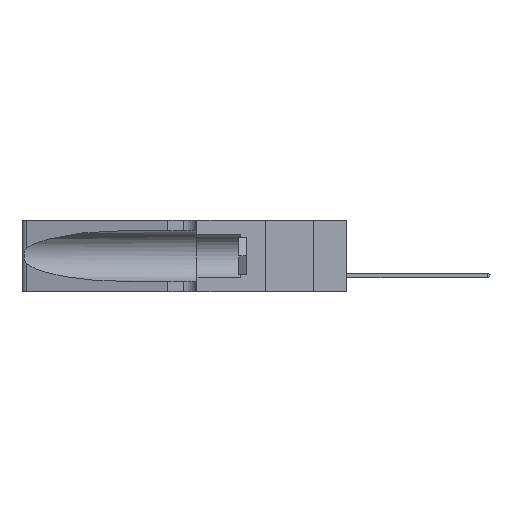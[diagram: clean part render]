
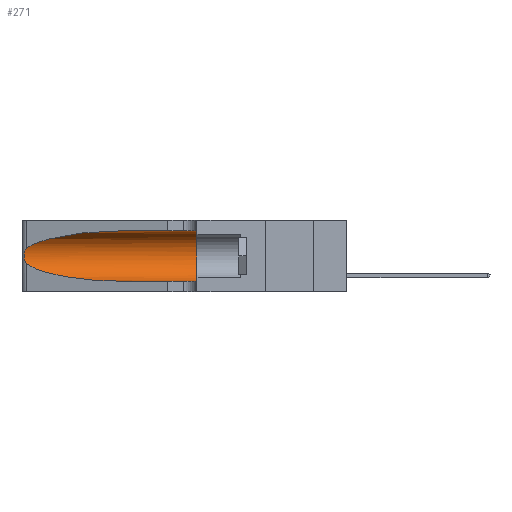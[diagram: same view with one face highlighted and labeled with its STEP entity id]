
A CAD part, left-side view. The second image highlights one B-rep face of the part: STEP entity #271.
In plain terms, the highlighted cylindrical face has radius 3.308 mm (diameter 6.617 mm), a partial arc.
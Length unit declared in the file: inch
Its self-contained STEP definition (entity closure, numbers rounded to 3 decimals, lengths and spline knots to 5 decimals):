
#271 = ADVANCED_FACE ( 'NONE', ( #20561 ), #32296, .F. ) ;
#334 = VERTEX_POINT ( 'NONE', #22993 ) ;
#437 = EDGE_LOOP ( 'NONE', ( #36061, #23964, #4984, #29937, #17057, #5986 ) ) ;
#499 = DIRECTION ( 'NONE',  ( 0., -1., 0. ) ) ;
#3479 = VERTEX_POINT ( 'NONE', #29351 ) ;
#3822 = LINE ( 'NONE', #5627, #8558 ) ;
#3956 = CARTESIAN_POINT ( 'NONE',  ( 0.26075, 1.23896, 0.178 ) ) ;
#3970 = CARTESIAN_POINT ( 'NONE',  ( 0.18966, 0.96281, 0.05475 ) ) ;
#4095 = CARTESIAN_POINT ( 'NONE',  ( 0.26075, 1.23896, 0.19203 ) ) ;
#4477 = CARTESIAN_POINT ( 'NONE',  ( 0.25487, 1.22718, 0.22369 ) ) ;
#4726 = EDGE_CURVE ( 'NONE', #3479, #27880, #16341, .T. ) ;
#4984 = ORIENTED_EDGE ( 'NONE', *, *, #6401, .T. ) ;
#5206 = VERTEX_POINT ( 'NONE', #27979 ) ;
#5441 = B_SPLINE_CURVE_WITH_KNOTS ( 'NONE', 3,
 ( #32488, #29800, #38594, #38480, #18253, #21294, #4095, #3956, #30803, #10031, #19609, #34381, #37412, #28608 ),
 .UNSPECIFIED., .F., .F.,
 ( 4, 2, 2, 2, 2, 2, 4 ),
 ( 0., 0.00027, 0.00053, 0.00107, 0.0016, 0.00187, 0.00214 ),
 .UNSPECIFIED. ) ;
#5627 = CARTESIAN_POINT ( 'NONE',  ( 0.1305, 1.61858, 0.31525 ) ) ;
#5986 = ORIENTED_EDGE ( 'NONE', *, *, #37150, .F. ) ;
#6135 = AXIS2_PLACEMENT_3D ( 'NONE', #24913, #18904, #18771 ) ;
#6401 = EDGE_CURVE ( 'NONE', #32020, #29624, #7006, .T. ) ;
#7006 =( BOUNDED_CURVE ( )  B_SPLINE_CURVE ( 3, ( #28217, #18804, #3970, #33987 ),
 .UNSPECIFIED., .F., .F. ) 
 B_SPLINE_CURVE_WITH_KNOTS ( ( 4, 4 ),
 ( 3.44316, 4.71239 ),
 .UNSPECIFIED. ) 
 CURVE ( )  GEOMETRIC_REPRESENTATION_ITEM ( )  RATIONAL_B_SPLINE_CURVE ( ( 1., 0.87, 0.87, 1. ) ) 
 REPRESENTATION_ITEM ( '' )  );
#7859 = CARTESIAN_POINT ( 'NONE',  ( 0.25487, 1.22718, 0.22369 ) ) ;
#8558 = VECTOR ( 'NONE', #35507, 39.37008 ) ;
#10031 = CARTESIAN_POINT ( 'NONE',  ( 0.25856, 1.23593, 0.16098 ) ) ;
#15086 = CARTESIAN_POINT ( 'NONE',  ( 0.1305, 1.61858, 0.185 ) ) ;
#15327 = DIRECTION ( 'NONE',  ( 0., 0., -1. ) ) ;
#16226 = CARTESIAN_POINT ( 'NONE',  ( 0.25487, 1.22718, 0.14631 ) ) ;
#16341 =( BOUNDED_CURVE ( )  B_SPLINE_CURVE ( 3, ( #28430, #34614, #19999, #7859 ),
 .UNSPECIFIED., .F., .F. ) 
 B_SPLINE_CURVE_WITH_KNOTS ( ( 4, 4 ),
 ( 1.5708, 2.84003 ),
 .UNSPECIFIED. ) 
 CURVE ( )  GEOMETRIC_REPRESENTATION_ITEM ( )  RATIONAL_B_SPLINE_CURVE ( ( 1., 0.87, 0.87, 1. ) ) 
 REPRESENTATION_ITEM ( '' )  );
#16529 = CARTESIAN_POINT ( 'NONE',  ( 0.1305, 0.72297, 0.05475 ) ) ;
#17057 = ORIENTED_EDGE ( 'NONE', *, *, #36085, .F. ) ;
#18253 = CARTESIAN_POINT ( 'NONE',  ( 0.25854, 1.2359, 0.20912 ) ) ;
#18771 = DIRECTION ( 'NONE',  ( 0., 0., 1. ) ) ;
#18804 = CARTESIAN_POINT ( 'NONE',  ( 0.2373, 1.15595, 0.08982 ) ) ;
#18904 = DIRECTION ( 'NONE',  ( 0., 1., 0. ) ) ;
#19235 = CIRCLE ( 'NONE', #6135, 0.13025 ) ;
#19609 = CARTESIAN_POINT ( 'NONE',  ( 0.25789, 1.23486, 0.15765 ) ) ;
#19999 = CARTESIAN_POINT ( 'NONE',  ( 0.2373, 1.15595, 0.28018 ) ) ;
#20561 = FACE_OUTER_BOUND ( 'NONE', #437, .T. ) ;
#21294 = CARTESIAN_POINT ( 'NONE',  ( 0.26018, 1.23835, 0.19895 ) ) ;
#22984 = VECTOR ( 'NONE', #36687, 39.37008 ) ;
#22993 = CARTESIAN_POINT ( 'NONE',  ( 0.1305, 0.35, 0.05475 ) ) ;
#23964 = ORIENTED_EDGE ( 'NONE', *, *, #24600, .T. ) ;
#24600 = EDGE_CURVE ( 'NONE', #27880, #32020, #5441, .T. ) ;
#24913 = CARTESIAN_POINT ( 'NONE',  ( 0.1305, 0.35, 0.185 ) ) ;
#27880 = VERTEX_POINT ( 'NONE', #4477 ) ;
#27979 = CARTESIAN_POINT ( 'NONE',  ( 0.1305, 0.35, 0.31525 ) ) ;
#28202 = AXIS2_PLACEMENT_3D ( 'NONE', #15086, #499, #15327 ) ;
#28217 = CARTESIAN_POINT ( 'NONE',  ( 0.25487, 1.22718, 0.14631 ) ) ;
#28430 = CARTESIAN_POINT ( 'NONE',  ( 0.1305, 0.72297, 0.31525 ) ) ;
#28608 = CARTESIAN_POINT ( 'NONE',  ( 0.25487, 1.22718, 0.14631 ) ) ;
#29351 = CARTESIAN_POINT ( 'NONE',  ( 0.1305, 0.72297, 0.31525 ) ) ;
#29624 = VERTEX_POINT ( 'NONE', #16529 ) ;
#29800 = CARTESIAN_POINT ( 'NONE',  ( 0.25555, 1.22994, 0.2215 ) ) ;
#29937 = ORIENTED_EDGE ( 'NONE', *, *, #31227, .T. ) ;
#30637 = CARTESIAN_POINT ( 'NONE',  ( 0.1305, 1.61858, 0.05475 ) ) ;
#30803 = CARTESIAN_POINT ( 'NONE',  ( 0.26017, 1.23833, 0.17102 ) ) ;
#31227 = EDGE_CURVE ( 'NONE', #29624, #334, #31912, .T. ) ;
#31912 = LINE ( 'NONE', #30637, #22984 ) ;
#32020 = VERTEX_POINT ( 'NONE', #16226 ) ;
#32296 = CYLINDRICAL_SURFACE ( 'NONE', #28202, 0.13025 ) ;
#32488 = CARTESIAN_POINT ( 'NONE',  ( 0.25487, 1.22718, 0.22369 ) ) ;
#33987 = CARTESIAN_POINT ( 'NONE',  ( 0.1305, 0.72297, 0.05475 ) ) ;
#34381 = CARTESIAN_POINT ( 'NONE',  ( 0.25639, 1.23186, 0.15144 ) ) ;
#34614 = CARTESIAN_POINT ( 'NONE',  ( 0.18966, 0.96281, 0.31525 ) ) ;
#35507 = DIRECTION ( 'NONE',  ( 0., -1., 0. ) ) ;
#36061 = ORIENTED_EDGE ( 'NONE', *, *, #4726, .T. ) ;
#36085 = EDGE_CURVE ( 'NONE', #5206, #334, #19235, .T. ) ;
#36687 = DIRECTION ( 'NONE',  ( 0., -1., 0. ) ) ;
#37150 = EDGE_CURVE ( 'NONE', #3479, #5206, #3822, .T. ) ;
#37412 = CARTESIAN_POINT ( 'NONE',  ( 0.25555, 1.22993, 0.14849 ) ) ;
#38480 = CARTESIAN_POINT ( 'NONE',  ( 0.25787, 1.23484, 0.2124 ) ) ;
#38594 = CARTESIAN_POINT ( 'NONE',  ( 0.25639, 1.23184, 0.21858 ) ) ;
